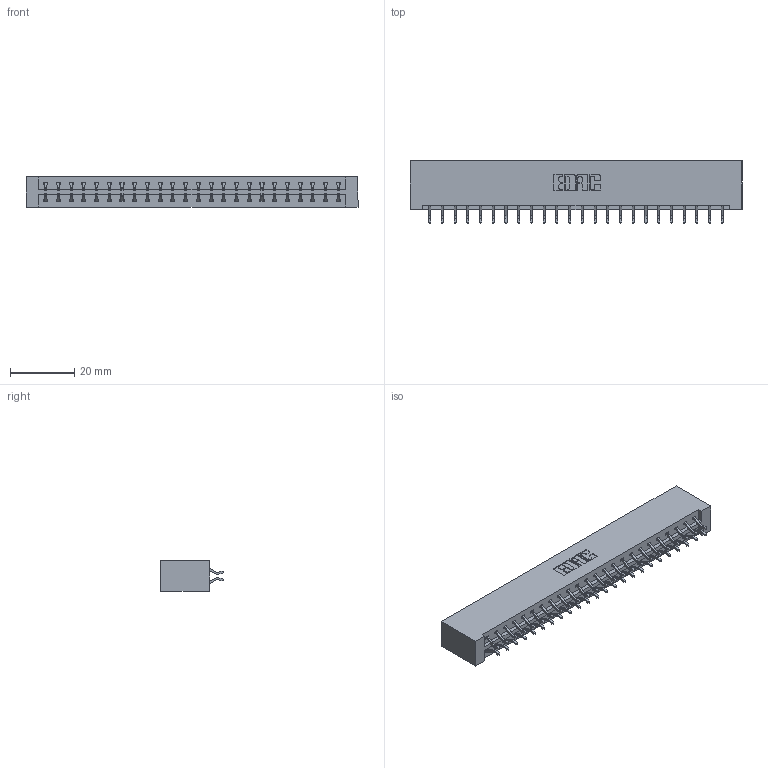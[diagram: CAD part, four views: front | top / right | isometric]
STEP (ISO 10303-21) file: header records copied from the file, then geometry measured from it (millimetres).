
FILE_DESCRIPTION (( 'STEP AP203' ), '1' );
FILE_NAME ('833-048-556-201.STEP', '2020-06-04T16:25:11', ( '' ), ( '' ), 'SwSTEP 2.0', 'SolidWorks 2020', '' );
FILE_SCHEMA (( 'CONFIG_CONTROL_DESIGN' ));
Length unit declared in the file: inch
Products named in the file (3): 345-292-001_556 Tail; 833 Part_Lugless; 833-048-556-201
Assembly tree (49 placements, depth 2):
  833-048-556-201
    833 Part_Lugless
    345-292-001_556 Tail  x48
Bounding box: 103.35 x 19.57 x 9.4 mm (x, y, z)
Volume: 11013.7 mm3; surface area: 12804.5 mm2
Topology: 49 solids, 49 shells, 2890 faces, 8591 edges, 5662 vertices
Faces by surface type: plane 1986, cylinder 904
Entity records: 17711 total; most frequent: CARTESIAN_POINT 2970, ORIENTED_EDGE 2894, DIRECTION 2551, EDGE_CURVE 1447, VECTOR 1319, LINE 1319, VERTEX_POINT 962, AXIS2_PLACEMENT_3D 616
